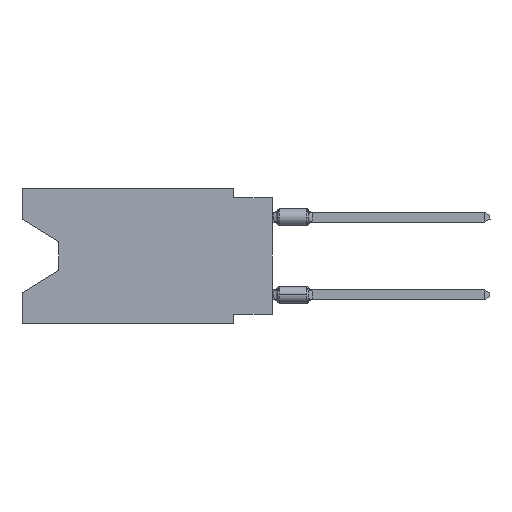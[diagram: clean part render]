
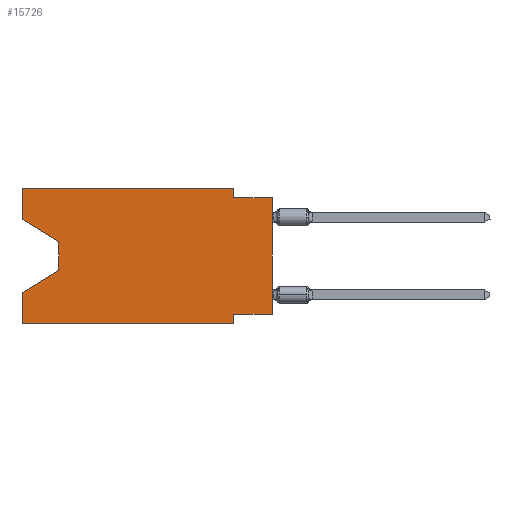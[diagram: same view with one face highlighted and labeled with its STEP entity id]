
A CAD part, left-side view. The second image highlights one B-rep face of the part: STEP entity #15726.
In plain terms, the highlighted planar face has unit normal (-1, 0, 0).
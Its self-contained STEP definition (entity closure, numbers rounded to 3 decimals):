
#235 = VERTEX_POINT ( 'NONE', #20182 ) ;
#371 = LINE ( 'NONE', #22967, #2716 ) ;
#956 = VERTEX_POINT ( 'NONE', #6962 ) ;
#2515 = CARTESIAN_POINT ( 'NONE',  ( 0., 13.97, -3.505 ) ) ;
#2560 = LINE ( 'NONE', #5702, #6702 ) ;
#2716 = VECTOR ( 'NONE', #30171, 1000. ) ;
#2769 = DIRECTION ( 'NONE',  ( 0., 0.855, -0.519 ) ) ;
#3023 = CARTESIAN_POINT ( 'NONE',  ( 0., 16.383, 0. ) ) ;
#4030 = VECTOR ( 'NONE', #43968, 1000. ) ;
#4301 = DIRECTION ( 'NONE',  ( 0., -0.855, -0.519 ) ) ;
#4522 = CARTESIAN_POINT ( 'NONE',  ( 0., 16.383, -6.852 ) ) ;
#4545 = ORIENTED_EDGE ( 'NONE', *, *, #47355, .F. ) ;
#5414 = EDGE_CURVE ( 'NONE', #39879, #46605, #41070, .T. ) ;
#5702 = CARTESIAN_POINT ( 'NONE',  ( 0., 2.54, -8.89 ) ) ;
#6702 = VECTOR ( 'NONE', #42942, 1000. ) ;
#6962 = CARTESIAN_POINT ( 'NONE',  ( 0., 0., -0.635 ) ) ;
#6983 = CARTESIAN_POINT ( 'NONE',  ( 0., 16.383, 0. ) ) ;
#7232 = DIRECTION ( 'NONE',  ( 0., 0., 1. ) ) ;
#7360 = ORIENTED_EDGE ( 'NONE', *, *, #18107, .F. ) ;
#7454 = DIRECTION ( 'NONE',  ( 0., 0., -1. ) ) ;
#7701 = LINE ( 'NONE', #3023, #29490 ) ;
#8526 = LINE ( 'NONE', #38300, #38764 ) ;
#10253 = VECTOR ( 'NONE', #14991, 1000. ) ;
#10683 = ORIENTED_EDGE ( 'NONE', *, *, #5414, .F. ) ;
#10802 = VERTEX_POINT ( 'NONE', #45880 ) ;
#10804 = ORIENTED_EDGE ( 'NONE', *, *, #35739, .T. ) ;
#11122 = DIRECTION ( 'NONE',  ( 1., 0., 0. ) ) ;
#11889 = LINE ( 'NONE', #41036, #45035 ) ;
#12042 = ORIENTED_EDGE ( 'NONE', *, *, #49086, .F. ) ;
#13332 = LINE ( 'NONE', #28961, #19968 ) ;
#14133 = PLANE ( 'NONE',  #27578 ) ;
#14159 = LINE ( 'NONE', #2515, #4030 ) ;
#14190 = LINE ( 'NONE', #6983, #19247 ) ;
#14850 = FACE_OUTER_BOUND ( 'NONE', #43126, .T. ) ;
#14991 = DIRECTION ( 'NONE',  ( 0., 1., 0. ) ) ;
#15382 = VECTOR ( 'NONE', #29492, 1000. ) ;
#15550 = VERTEX_POINT ( 'NONE', #4522 ) ;
#15726 = ADVANCED_FACE ( 'NONE', ( #14850 ), #14133, .F. ) ;
#16004 = VECTOR ( 'NONE', #7454, 1000. ) ;
#16632 = VERTEX_POINT ( 'NONE', #18219 ) ;
#18107 = EDGE_CURVE ( 'NONE', #44114, #956, #11889, .T. ) ;
#18219 = CARTESIAN_POINT ( 'NONE',  ( 0., 2.54, -8.89 ) ) ;
#18469 = ORIENTED_EDGE ( 'NONE', *, *, #36994, .F. ) ;
#19180 = CARTESIAN_POINT ( 'NONE',  ( 0., 0., -8.255 ) ) ;
#19247 = VECTOR ( 'NONE', #44951, 1000. ) ;
#19968 = VECTOR ( 'NONE', #32458, 1000. ) ;
#20182 = CARTESIAN_POINT ( 'NONE',  ( 0., 13.97, -3.505 ) ) ;
#20278 = ORIENTED_EDGE ( 'NONE', *, *, #32411, .T. ) ;
#22967 = CARTESIAN_POINT ( 'NONE',  ( 0., 0., 0. ) ) ;
#22983 = VERTEX_POINT ( 'NONE', #36960 ) ;
#23063 = CARTESIAN_POINT ( 'NONE',  ( 0., 0., -8.255 ) ) ;
#23521 = EDGE_CURVE ( 'NONE', #39879, #956, #371, .T. ) ;
#25799 = DIRECTION ( 'NONE',  ( 0., 0., -1. ) ) ;
#25860 = LINE ( 'NONE', #29817, #16004 ) ;
#26149 = DIRECTION ( 'NONE',  ( 0., -1., 0. ) ) ;
#27063 = ORIENTED_EDGE ( 'NONE', *, *, #37056, .F. ) ;
#27578 = AXIS2_PLACEMENT_3D ( 'NONE', #37219, #11122, #25799 ) ;
#28097 = VERTEX_POINT ( 'NONE', #30833 ) ;
#28256 = ORIENTED_EDGE ( 'NONE', *, *, #44863, .T. ) ;
#28961 = CARTESIAN_POINT ( 'NONE',  ( 0., 16.383, -8.89 ) ) ;
#29490 = VECTOR ( 'NONE', #7232, 1000. ) ;
#29492 = DIRECTION ( 'NONE',  ( 0., 0., 1. ) ) ;
#29808 = CARTESIAN_POINT ( 'NONE',  ( 0., 13.97, -5.385 ) ) ;
#29817 = CARTESIAN_POINT ( 'NONE',  ( 0., 2.54, 0. ) ) ;
#30136 = VERTEX_POINT ( 'NONE', #31861 ) ;
#30171 = DIRECTION ( 'NONE',  ( 0., 0., 1. ) ) ;
#30833 = CARTESIAN_POINT ( 'NONE',  ( 0., 16.383, -2.038 ) ) ;
#31781 = ORIENTED_EDGE ( 'NONE', *, *, #23521, .T. ) ;
#31861 = CARTESIAN_POINT ( 'NONE',  ( 0., 16.383, -8.89 ) ) ;
#32411 = EDGE_CURVE ( 'NONE', #28097, #235, #8526, .T. ) ;
#32458 = DIRECTION ( 'NONE',  ( 0., -1., 0. ) ) ;
#32730 = CARTESIAN_POINT ( 'NONE',  ( 0., 2.54, -0.635 ) ) ;
#33219 = LINE ( 'NONE', #47657, #15382 ) ;
#33299 = LINE ( 'NONE', #29808, #46065 ) ;
#35254 = CARTESIAN_POINT ( 'NONE',  ( 0., 16.383, 0. ) ) ;
#35739 = EDGE_CURVE ( 'NONE', #10802, #15550, #33299, .T. ) ;
#36960 = CARTESIAN_POINT ( 'NONE',  ( 0., 2.54, 0. ) ) ;
#36994 = EDGE_CURVE ( 'NONE', #22983, #44114, #25860, .T. ) ;
#37056 = EDGE_CURVE ( 'NONE', #30136, #15550, #7701, .T. ) ;
#37061 = ORIENTED_EDGE ( 'NONE', *, *, #40255, .F. ) ;
#37219 = CARTESIAN_POINT ( 'NONE',  ( 0., 16.383, 0. ) ) ;
#37497 = EDGE_CURVE ( 'NONE', #30136, #16632, #13332, .T. ) ;
#38300 = CARTESIAN_POINT ( 'NONE',  ( 0., 16.383, -2.038 ) ) ;
#38764 = VECTOR ( 'NONE', #4301, 1000. ) ;
#39879 = VERTEX_POINT ( 'NONE', #23063 ) ;
#40255 = EDGE_CURVE ( 'NONE', #28097, #43518, #33219, .T. ) ;
#41036 = CARTESIAN_POINT ( 'NONE',  ( 0., 0., -0.635 ) ) ;
#41070 = LINE ( 'NONE', #19180, #10253 ) ;
#41408 = CARTESIAN_POINT ( 'NONE',  ( 0., 2.54, -8.255 ) ) ;
#42790 = ORIENTED_EDGE ( 'NONE', *, *, #37497, .T. ) ;
#42942 = DIRECTION ( 'NONE',  ( 0., 0., -1. ) ) ;
#43126 = EDGE_LOOP ( 'NONE', ( #20278, #28256, #10804, #27063, #42790, #12042, #10683, #31781, #7360, #18469, #4545, #37061 ) ) ;
#43518 = VERTEX_POINT ( 'NONE', #35254 ) ;
#43968 = DIRECTION ( 'NONE',  ( 0., 0., -1. ) ) ;
#44114 = VERTEX_POINT ( 'NONE', #32730 ) ;
#44863 = EDGE_CURVE ( 'NONE', #235, #10802, #14159, .T. ) ;
#44951 = DIRECTION ( 'NONE',  ( 0., -1., 0. ) ) ;
#45035 = VECTOR ( 'NONE', #26149, 1000. ) ;
#45880 = CARTESIAN_POINT ( 'NONE',  ( 0., 13.97, -5.385 ) ) ;
#46065 = VECTOR ( 'NONE', #2769, 1000. ) ;
#46605 = VERTEX_POINT ( 'NONE', #41408 ) ;
#47355 = EDGE_CURVE ( 'NONE', #43518, #22983, #14190, .T. ) ;
#47657 = CARTESIAN_POINT ( 'NONE',  ( 0., 16.383, 0. ) ) ;
#49086 = EDGE_CURVE ( 'NONE', #46605, #16632, #2560, .T. ) ;
